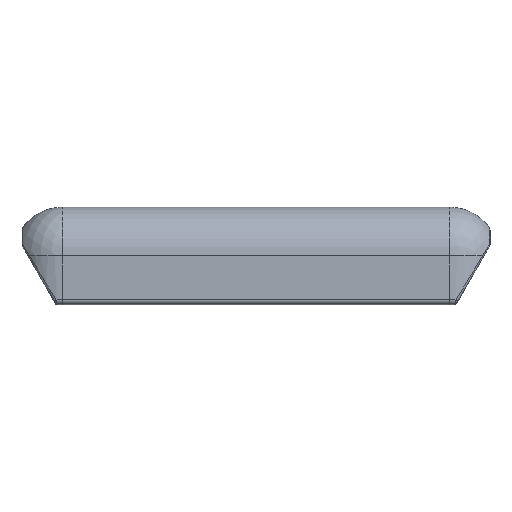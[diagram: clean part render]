
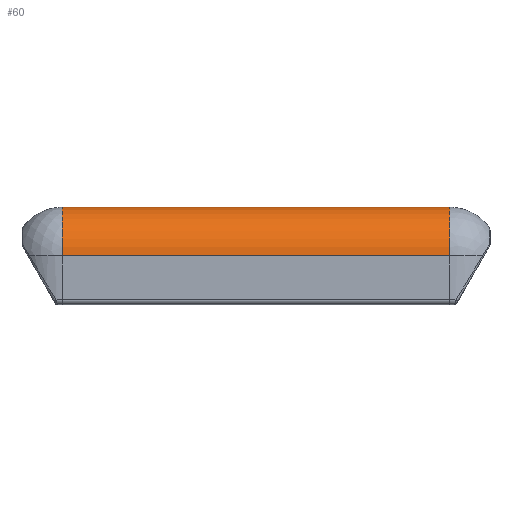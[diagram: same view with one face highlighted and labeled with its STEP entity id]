
A CAD part, top view. The second image highlights one B-rep face of the part: STEP entity #60.
In plain terms, the highlighted cylindrical face has radius 10 mm (diameter 20 mm), a partial arc.
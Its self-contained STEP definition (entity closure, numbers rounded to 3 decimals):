
#23 = CARTESIAN_POINT ( 'NONE',  ( -352.19, 43.089, 4.723 ) ) ;
#34 = DIRECTION ( 'NONE',  ( 1., 0., 0. ) ) ;
#60 = ADVANCED_FACE ( 'NONE', ( #1976 ), #2018, .T. ) ;
#167 = CARTESIAN_POINT ( 'NONE',  ( -431.634, 53.089, 4.723 ) ) ;
#210 = CARTESIAN_POINT ( 'NONE',  ( -352.19, 53.089, 4.723 ) ) ;
#342 = AXIS2_PLACEMENT_3D ( 'NONE', #3165, #34, #2753 ) ;
#550 = AXIS2_PLACEMENT_3D ( 'NONE', #1681, #1908, #2151 ) ;
#584 = VERTEX_POINT ( 'NONE', #167 ) ;
#608 = LINE ( 'NONE', #2220, #900 ) ;
#624 = VERTEX_POINT ( 'NONE', #3257 ) ;
#625 = CIRCLE ( 'NONE', #342, 10. ) ;
#878 = EDGE_CURVE ( 'NONE', #624, #2503, #608, .T. ) ;
#900 = VECTOR ( 'NONE', #932, 1000. ) ;
#932 = DIRECTION ( 'NONE',  ( 1., 0., 0. ) ) ;
#952 = LINE ( 'NONE', #1347, #2652 ) ;
#1091 = DIRECTION ( 'NONE',  ( -1., 0., 0. ) ) ;
#1261 = EDGE_CURVE ( 'NONE', #2917, #584, #952, .T. ) ;
#1347 = CARTESIAN_POINT ( 'NONE',  ( -391.535, 53.089, 4.723 ) ) ;
#1350 = CIRCLE ( 'NONE', #1472, 10. ) ;
#1454 = ORIENTED_EDGE ( 'NONE', *, *, #1553, .T. ) ;
#1472 = AXIS2_PLACEMENT_3D ( 'NONE', #23, #2373, #2863 ) ;
#1553 = EDGE_CURVE ( 'NONE', #584, #624, #625, .T. ) ;
#1654 = ORIENTED_EDGE ( 'NONE', *, *, #878, .T. ) ;
#1681 = CARTESIAN_POINT ( 'NONE',  ( -391.535, 43.089, 4.723 ) ) ;
#1908 = DIRECTION ( 'NONE',  ( -1., 0., 0. ) ) ;
#1976 = FACE_OUTER_BOUND ( 'NONE', #2304, .T. ) ;
#2018 = CYLINDRICAL_SURFACE ( 'NONE', #550, 10. ) ;
#2151 = DIRECTION ( 'NONE',  ( 0., 0.707, 0.707 ) ) ;
#2220 = CARTESIAN_POINT ( 'NONE',  ( -391.535, 43.089, 14.723 ) ) ;
#2304 = EDGE_LOOP ( 'NONE', ( #3215, #3006, #1454, #1654 ) ) ;
#2373 = DIRECTION ( 'NONE',  ( -1., 0., 0. ) ) ;
#2503 = VERTEX_POINT ( 'NONE', #2603 ) ;
#2603 = CARTESIAN_POINT ( 'NONE',  ( -352.19, 43.089, 14.723 ) ) ;
#2652 = VECTOR ( 'NONE', #1091, 1000. ) ;
#2753 = DIRECTION ( 'NONE',  ( 0., 1., 0. ) ) ;
#2863 = DIRECTION ( 'NONE',  ( 0., 0., 1. ) ) ;
#2917 = VERTEX_POINT ( 'NONE', #210 ) ;
#3006 = ORIENTED_EDGE ( 'NONE', *, *, #1261, .T. ) ;
#3013 = EDGE_CURVE ( 'NONE', #2503, #2917, #1350, .T. ) ;
#3165 = CARTESIAN_POINT ( 'NONE',  ( -431.634, 43.089, 4.723 ) ) ;
#3215 = ORIENTED_EDGE ( 'NONE', *, *, #3013, .T. ) ;
#3257 = CARTESIAN_POINT ( 'NONE',  ( -431.634, 43.089, 14.723 ) ) ;
